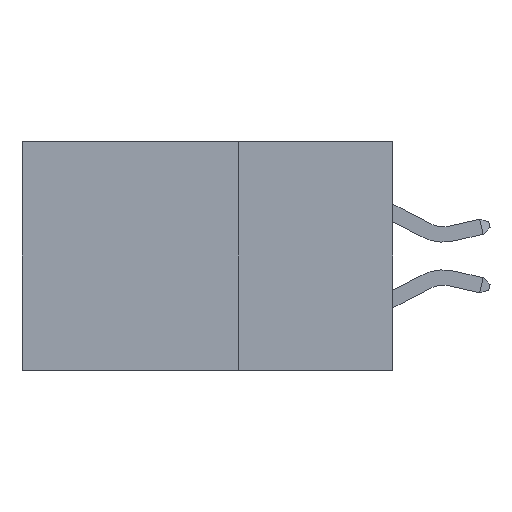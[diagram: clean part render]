
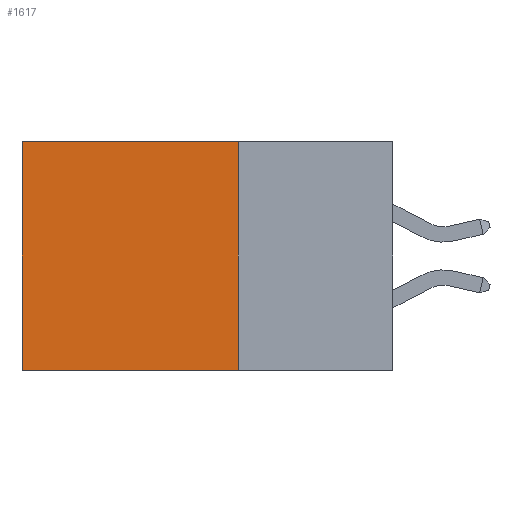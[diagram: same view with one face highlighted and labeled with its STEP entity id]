
A CAD part, left-side view. The second image highlights one B-rep face of the part: STEP entity #1617.
In plain terms, the highlighted planar face has unit normal (-1, 0, 0).
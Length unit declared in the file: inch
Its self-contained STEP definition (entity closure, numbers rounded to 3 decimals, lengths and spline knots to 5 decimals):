
#86 = EDGE_CURVE ( 'NONE', #586, #12035, #8051, .T. ) ;
#317 = EDGE_CURVE ( 'NONE', #14096, #29133, #21455, .T. ) ;
#586 = VERTEX_POINT ( 'NONE', #28620 ) ;
#1617 = ADVANCED_FACE ( 'NONE', ( #14013 ), #20862, .F. ) ;
#2632 = EDGE_CURVE ( 'NONE', #29133, #12035, #15111, .T. ) ;
#3133 = ORIENTED_EDGE ( 'NONE', *, *, #86, .T. ) ;
#3568 = CARTESIAN_POINT ( 'NONE',  ( 0.2875, 0.25, 0. ) ) ;
#6609 = CARTESIAN_POINT ( 'NONE',  ( 0.2875, 0.25, -0.37 ) ) ;
#6962 = EDGE_LOOP ( 'NONE', ( #3133, #9870, #21852, #30631 ) ) ;
#7158 = DIRECTION ( 'NONE',  ( 0., 0., -1. ) ) ;
#7405 = CARTESIAN_POINT ( 'NONE',  ( 0.2875, 0.25, 0. ) ) ;
#7655 = VECTOR ( 'NONE', #18319, 39.37008 ) ;
#8051 = LINE ( 'NONE', #22869, #7655 ) ;
#8099 = AXIS2_PLACEMENT_3D ( 'NONE', #23354, #28093, #18160 ) ;
#9650 = CARTESIAN_POINT ( 'NONE',  ( 0.2875, 0.25, -0.37 ) ) ;
#9870 = ORIENTED_EDGE ( 'NONE', *, *, #2632, .F. ) ;
#11656 = VECTOR ( 'NONE', #15783, 39.37008 ) ;
#12035 = VERTEX_POINT ( 'NONE', #30840 ) ;
#12771 = LINE ( 'NONE', #3568, #11656 ) ;
#14013 = FACE_OUTER_BOUND ( 'NONE', #6962, .T. ) ;
#14096 = VERTEX_POINT ( 'NONE', #7405 ) ;
#15111 = LINE ( 'NONE', #6609, #30195 ) ;
#15783 = DIRECTION ( 'NONE',  ( 0., 1., 0. ) ) ;
#18160 = DIRECTION ( 'NONE',  ( 0., 0., -1. ) ) ;
#18319 = DIRECTION ( 'NONE',  ( 0., 0., -1. ) ) ;
#20862 = PLANE ( 'NONE',  #8099 ) ;
#21455 = LINE ( 'NONE', #23622, #23423 ) ;
#21852 = ORIENTED_EDGE ( 'NONE', *, *, #317, .F. ) ;
#22869 = CARTESIAN_POINT ( 'NONE',  ( 0.2875, 0.6, 0. ) ) ;
#23354 = CARTESIAN_POINT ( 'NONE',  ( 0.2875, 0.25, 0. ) ) ;
#23423 = VECTOR ( 'NONE', #7158, 39.37008 ) ;
#23622 = CARTESIAN_POINT ( 'NONE',  ( 0.2875, 0.25, 0. ) ) ;
#27566 = EDGE_CURVE ( 'NONE', #14096, #586, #12771, .T. ) ;
#28093 = DIRECTION ( 'NONE',  ( 1., 0., 0. ) ) ;
#28620 = CARTESIAN_POINT ( 'NONE',  ( 0.2875, 0.6, 0. ) ) ;
#29133 = VERTEX_POINT ( 'NONE', #9650 ) ;
#30195 = VECTOR ( 'NONE', #31675, 39.37008 ) ;
#30631 = ORIENTED_EDGE ( 'NONE', *, *, #27566, .T. ) ;
#30840 = CARTESIAN_POINT ( 'NONE',  ( 0.2875, 0.6, -0.37 ) ) ;
#31675 = DIRECTION ( 'NONE',  ( 0., 1., 0. ) ) ;
